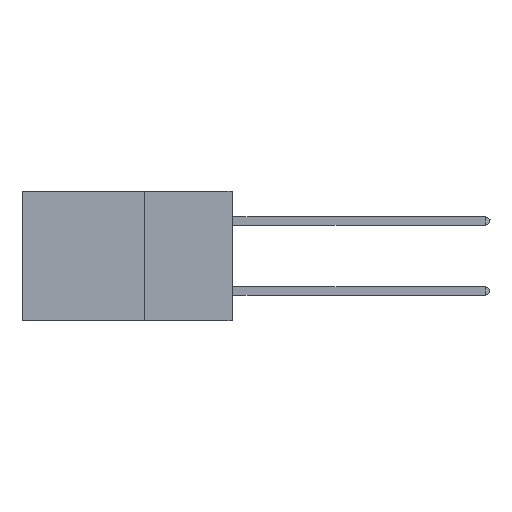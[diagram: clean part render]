
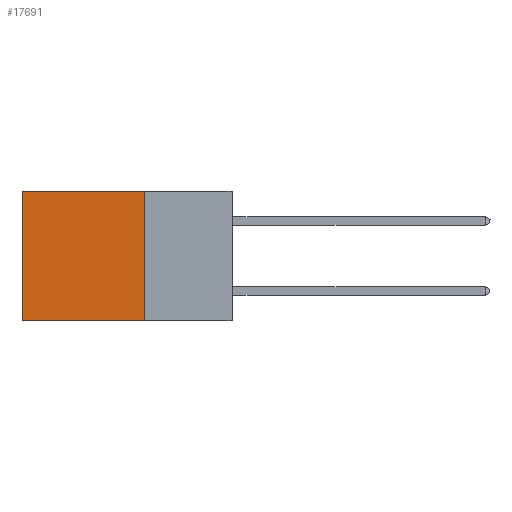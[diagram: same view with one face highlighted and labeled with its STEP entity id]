
A CAD part, left-side view. The second image highlights one B-rep face of the part: STEP entity #17691.
In plain terms, the highlighted planar face has unit normal (-1, 0, 0).
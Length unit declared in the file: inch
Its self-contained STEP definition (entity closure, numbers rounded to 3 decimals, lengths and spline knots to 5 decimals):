
#76 = DIRECTION ( 'NONE',  ( 0., 0., -1. ) ) ;
#210 = EDGE_CURVE ( 'NONE', #11564, #3323, #7919, .T. ) ;
#665 = PLANE ( 'NONE',  #2203 ) ;
#794 = EDGE_CURVE ( 'NONE', #5077, #11564, #16624, .T. ) ;
#1239 = CARTESIAN_POINT ( 'NONE',  ( 0.2875, 0.6, -0.37 ) ) ;
#2203 = AXIS2_PLACEMENT_3D ( 'NONE', #11963, #13431, #2256 ) ;
#2256 = DIRECTION ( 'NONE',  ( 0., 0., -1. ) ) ;
#2753 = ORIENTED_EDGE ( 'NONE', *, *, #8008, .T. ) ;
#2918 = VECTOR ( 'NONE', #16726, 39.37008 ) ;
#3323 = VERTEX_POINT ( 'NONE', #1239 ) ;
#3915 = CARTESIAN_POINT ( 'NONE',  ( 0.2875, 0.6, 0. ) ) ;
#4143 = VECTOR ( 'NONE', #17618, 39.37008 ) ;
#5077 = VERTEX_POINT ( 'NONE', #17996 ) ;
#6690 = ORIENTED_EDGE ( 'NONE', *, *, #210, .F. ) ;
#7088 = ORIENTED_EDGE ( 'NONE', *, *, #18663, .T. ) ;
#7362 = CARTESIAN_POINT ( 'NONE',  ( 0.2875, 0.6, 0. ) ) ;
#7919 = LINE ( 'NONE', #17729, #4143 ) ;
#8008 = EDGE_CURVE ( 'NONE', #5077, #8152, #13080, .T. ) ;
#8152 = VERTEX_POINT ( 'NONE', #3915 ) ;
#11564 = VERTEX_POINT ( 'NONE', #16323 ) ;
#11603 = VECTOR ( 'NONE', #14557, 39.37008 ) ;
#11963 = CARTESIAN_POINT ( 'NONE',  ( 0.2875, 0.25, 0. ) ) ;
#12250 = EDGE_LOOP ( 'NONE', ( #7088, #6690, #20720, #2753 ) ) ;
#13080 = LINE ( 'NONE', #17941, #11603 ) ;
#13361 = CARTESIAN_POINT ( 'NONE',  ( 0.2875, 0.25, 0. ) ) ;
#13431 = DIRECTION ( 'NONE',  ( 1., 0., 0. ) ) ;
#13534 = FACE_OUTER_BOUND ( 'NONE', #12250, .T. ) ;
#14557 = DIRECTION ( 'NONE',  ( 0., 1., 0. ) ) ;
#16323 = CARTESIAN_POINT ( 'NONE',  ( 0.2875, 0.25, -0.37 ) ) ;
#16624 = LINE ( 'NONE', #13361, #18612 ) ;
#16726 = DIRECTION ( 'NONE',  ( 0., 0., -1. ) ) ;
#17618 = DIRECTION ( 'NONE',  ( 0., 1., 0. ) ) ;
#17691 = ADVANCED_FACE ( 'NONE', ( #13534 ), #665, .F. ) ;
#17729 = CARTESIAN_POINT ( 'NONE',  ( 0.2875, 0.25, -0.37 ) ) ;
#17941 = CARTESIAN_POINT ( 'NONE',  ( 0.2875, 0.25, 0. ) ) ;
#17996 = CARTESIAN_POINT ( 'NONE',  ( 0.2875, 0.25, 0. ) ) ;
#18330 = LINE ( 'NONE', #7362, #2918 ) ;
#18612 = VECTOR ( 'NONE', #76, 39.37008 ) ;
#18663 = EDGE_CURVE ( 'NONE', #8152, #3323, #18330, .T. ) ;
#20720 = ORIENTED_EDGE ( 'NONE', *, *, #794, .F. ) ;
